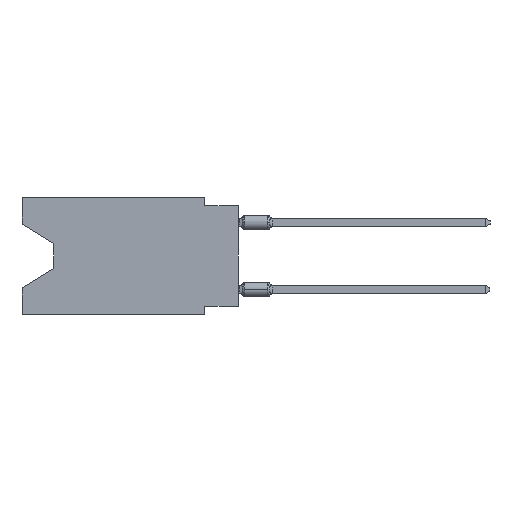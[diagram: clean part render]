
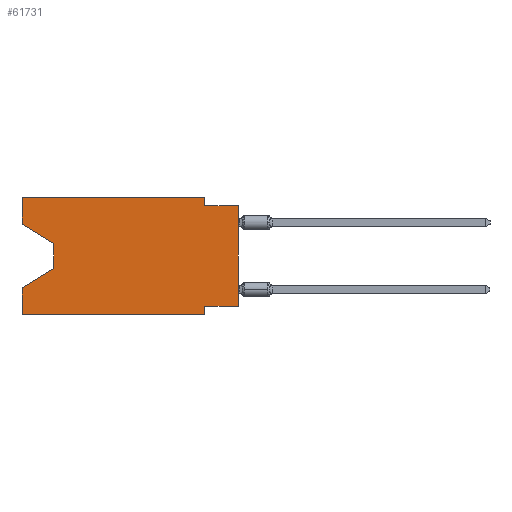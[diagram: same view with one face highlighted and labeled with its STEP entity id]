
A CAD part, left-side view. The second image highlights one B-rep face of the part: STEP entity #61731.
In plain terms, the highlighted planar face has unit normal (-1, 0, 0).
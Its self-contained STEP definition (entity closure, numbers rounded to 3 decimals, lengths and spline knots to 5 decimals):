
#368 = DIRECTION ( 'NONE',  ( 0., 0., 1. ) ) ;
#669 = EDGE_CURVE ( 'NONE', #30534, #39885, #15971, .T. ) ;
#702 = CARTESIAN_POINT ( 'NONE',  ( 0., 0.645, 0. ) ) ;
#807 = VERTEX_POINT ( 'NONE', #32481 ) ;
#4034 = EDGE_CURVE ( 'NONE', #7590, #14661, #57566, .T. ) ;
#4241 = CARTESIAN_POINT ( 'NONE',  ( 0., 0.645, -0.08025 ) ) ;
#5053 = CARTESIAN_POINT ( 'NONE',  ( 0., 0.645, 0. ) ) ;
#5059 = ORIENTED_EDGE ( 'NONE', *, *, #4034, .F. ) ;
#6445 = CARTESIAN_POINT ( 'NONE',  ( 0., 0.645, -0.26975 ) ) ;
#6721 = EDGE_CURVE ( 'NONE', #30534, #15607, #63614, .T. ) ;
#7160 = CARTESIAN_POINT ( 'NONE',  ( 0., 0.55, -0.138 ) ) ;
#7590 = VERTEX_POINT ( 'NONE', #54032 ) ;
#7771 = VERTEX_POINT ( 'NONE', #44607 ) ;
#7907 = EDGE_CURVE ( 'NONE', #55208, #11194, #42311, .T. ) ;
#8679 = CARTESIAN_POINT ( 'NONE',  ( 0., 0.645, 0. ) ) ;
#9521 = VECTOR ( 'NONE', #56475, 39.37008 ) ;
#10227 = EDGE_CURVE ( 'NONE', #14661, #15607, #52942, .T. ) ;
#10690 = DIRECTION ( 'NONE',  ( 0., -1., 0. ) ) ;
#11194 = VERTEX_POINT ( 'NONE', #54404 ) ;
#13280 = CARTESIAN_POINT ( 'NONE',  ( 0., 0.1, -0.025 ) ) ;
#13901 = VERTEX_POINT ( 'NONE', #19479 ) ;
#14661 = VERTEX_POINT ( 'NONE', #32643 ) ;
#15051 = EDGE_CURVE ( 'NONE', #807, #18088, #42889, .T. ) ;
#15607 = VERTEX_POINT ( 'NONE', #23763 ) ;
#15971 = LINE ( 'NONE', #702, #45443 ) ;
#16539 = EDGE_CURVE ( 'NONE', #7771, #37313, #63211, .T. ) ;
#17768 = DIRECTION ( 'NONE',  ( 1., 0., 0. ) ) ;
#18088 = VERTEX_POINT ( 'NONE', #18481 ) ;
#18230 = DIRECTION ( 'NONE',  ( 0., 0., -1. ) ) ;
#18481 = CARTESIAN_POINT ( 'NONE',  ( 0., 0.55, -0.212 ) ) ;
#18740 = CARTESIAN_POINT ( 'NONE',  ( 0., 0.645, 0. ) ) ;
#19479 = CARTESIAN_POINT ( 'NONE',  ( 0., 0.645, -0.08025 ) ) ;
#19558 = VECTOR ( 'NONE', #31572, 39.37008 ) ;
#20097 = CARTESIAN_POINT ( 'NONE',  ( 0., 0.645, -0.35 ) ) ;
#21406 = LINE ( 'NONE', #32753, #56879 ) ;
#22361 = DIRECTION ( 'NONE',  ( 0., 0., 1. ) ) ;
#22802 = VECTOR ( 'NONE', #59617, 39.37008 ) ;
#23087 = CARTESIAN_POINT ( 'NONE',  ( 0., 0.1, -0.35 ) ) ;
#23441 = ORIENTED_EDGE ( 'NONE', *, *, #10227, .F. ) ;
#23763 = CARTESIAN_POINT ( 'NONE',  ( 0., 0.1, -0.35 ) ) ;
#23789 = DIRECTION ( 'NONE',  ( 0., 1., 0. ) ) ;
#25340 = ORIENTED_EDGE ( 'NONE', *, *, #6721, .T. ) ;
#26412 = EDGE_LOOP ( 'NONE', ( #34350, #45792, #59025, #45024, #25340, #23441, #5059, #54276, #37458, #29437, #41675, #31406 ) ) ;
#28102 = CARTESIAN_POINT ( 'NONE',  ( 0., 0.645, -0.35 ) ) ;
#28485 = VECTOR ( 'NONE', #38055, 39.37008 ) ;
#28612 = LINE ( 'NONE', #4241, #28485 ) ;
#29210 = EDGE_CURVE ( 'NONE', #13901, #807, #28612, .T. ) ;
#29437 = ORIENTED_EDGE ( 'NONE', *, *, #45418, .F. ) ;
#30534 = VERTEX_POINT ( 'NONE', #28102 ) ;
#31406 = ORIENTED_EDGE ( 'NONE', *, *, #47722, .F. ) ;
#31572 = DIRECTION ( 'NONE',  ( 0., 0., -1. ) ) ;
#32481 = CARTESIAN_POINT ( 'NONE',  ( 0., 0.55, -0.138 ) ) ;
#32643 = CARTESIAN_POINT ( 'NONE',  ( 0., 0.1, -0.325 ) ) ;
#32753 = CARTESIAN_POINT ( 'NONE',  ( 0., 0., 0. ) ) ;
#34350 = ORIENTED_EDGE ( 'NONE', *, *, #29210, .T. ) ;
#36769 = LINE ( 'NONE', #37081, #19558 ) ;
#37010 = LINE ( 'NONE', #51291, #9521 ) ;
#37081 = CARTESIAN_POINT ( 'NONE',  ( 0., 0.1, 0. ) ) ;
#37313 = VERTEX_POINT ( 'NONE', #55865 ) ;
#37458 = ORIENTED_EDGE ( 'NONE', *, *, #7907, .F. ) ;
#37772 = CARTESIAN_POINT ( 'NONE',  ( 0., 0., -0.025 ) ) ;
#37993 = VECTOR ( 'NONE', #38555, 39.37008 ) ;
#38055 = DIRECTION ( 'NONE',  ( 0., -0.855, -0.519 ) ) ;
#38555 = DIRECTION ( 'NONE',  ( 0., -1., 0. ) ) ;
#39885 = VERTEX_POINT ( 'NONE', #6445 ) ;
#41675 = ORIENTED_EDGE ( 'NONE', *, *, #16539, .F. ) ;
#42311 = LINE ( 'NONE', #37772, #49779 ) ;
#42779 = DIRECTION ( 'NONE',  ( 0., 0., -1. ) ) ;
#42889 = LINE ( 'NONE', #7160, #57529 ) ;
#44607 = CARTESIAN_POINT ( 'NONE',  ( 0., 0.645, 0. ) ) ;
#45024 = ORIENTED_EDGE ( 'NONE', *, *, #669, .F. ) ;
#45418 = EDGE_CURVE ( 'NONE', #37313, #55208, #36769, .T. ) ;
#45443 = VECTOR ( 'NONE', #368, 39.37008 ) ;
#45792 = ORIENTED_EDGE ( 'NONE', *, *, #15051, .T. ) ;
#46206 = DIRECTION ( 'NONE',  ( 0., -1., 0. ) ) ;
#47722 = EDGE_CURVE ( 'NONE', #13901, #7771, #49539, .T. ) ;
#47838 = VECTOR ( 'NONE', #23789, 39.37008 ) ;
#48083 = DIRECTION ( 'NONE',  ( 0., 0., -1. ) ) ;
#49539 = LINE ( 'NONE', #5053, #22802 ) ;
#49600 = EDGE_CURVE ( 'NONE', #18088, #39885, #37010, .T. ) ;
#49779 = VECTOR ( 'NONE', #46206, 39.37008 ) ;
#49844 = VECTOR ( 'NONE', #48083, 39.37008 ) ;
#51291 = CARTESIAN_POINT ( 'NONE',  ( 0., 0.55, -0.212 ) ) ;
#52942 = LINE ( 'NONE', #23087, #49844 ) ;
#53000 = CARTESIAN_POINT ( 'NONE',  ( 0., 0., -0.325 ) ) ;
#53149 = FACE_OUTER_BOUND ( 'NONE', #26412, .T. ) ;
#53206 = EDGE_CURVE ( 'NONE', #7590, #11194, #21406, .T. ) ;
#54032 = CARTESIAN_POINT ( 'NONE',  ( 0., 0., -0.325 ) ) ;
#54276 = ORIENTED_EDGE ( 'NONE', *, *, #53206, .T. ) ;
#54404 = CARTESIAN_POINT ( 'NONE',  ( 0., 0., -0.025 ) ) ;
#55208 = VERTEX_POINT ( 'NONE', #13280 ) ;
#55865 = CARTESIAN_POINT ( 'NONE',  ( 0., 0.1, 0. ) ) ;
#56475 = DIRECTION ( 'NONE',  ( 0., 0.855, -0.519 ) ) ;
#56879 = VECTOR ( 'NONE', #22361, 39.37008 ) ;
#57368 = PLANE ( 'NONE',  #59446 ) ;
#57529 = VECTOR ( 'NONE', #18230, 39.37008 ) ;
#57566 = LINE ( 'NONE', #53000, #47838 ) ;
#58703 = VECTOR ( 'NONE', #10690, 39.37008 ) ;
#59025 = ORIENTED_EDGE ( 'NONE', *, *, #49600, .T. ) ;
#59446 = AXIS2_PLACEMENT_3D ( 'NONE', #8679, #17768, #42779 ) ;
#59617 = DIRECTION ( 'NONE',  ( 0., 0., 1. ) ) ;
#61731 = ADVANCED_FACE ( 'NONE', ( #53149 ), #57368, .F. ) ;
#63211 = LINE ( 'NONE', #18740, #37993 ) ;
#63614 = LINE ( 'NONE', #20097, #58703 ) ;
